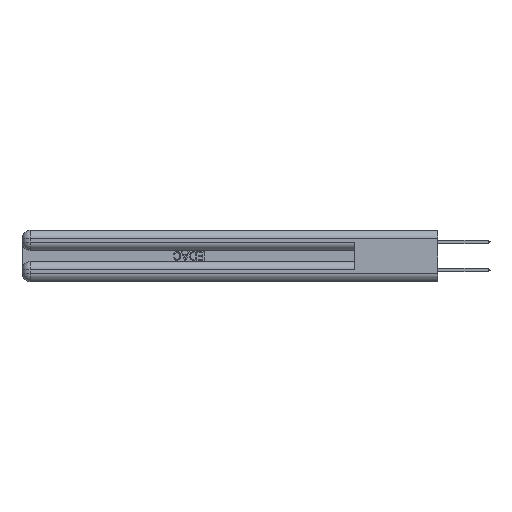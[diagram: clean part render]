
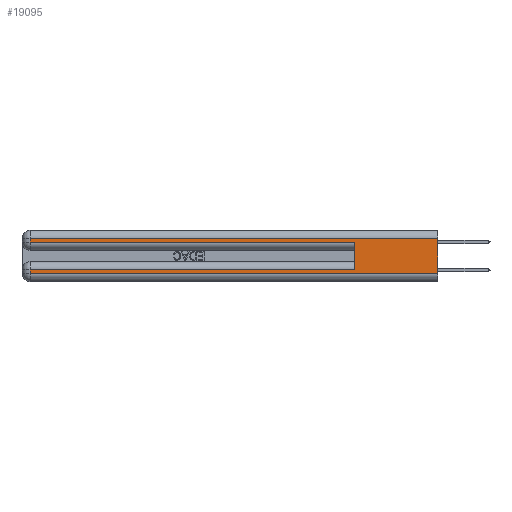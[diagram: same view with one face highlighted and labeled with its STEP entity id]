
A CAD part, left-side view. The second image highlights one B-rep face of the part: STEP entity #19095.
In plain terms, the highlighted planar face has unit normal (-1, 0, 0).
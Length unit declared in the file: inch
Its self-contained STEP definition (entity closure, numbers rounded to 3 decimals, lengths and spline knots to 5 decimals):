
#151 = DIRECTION ( 'NONE',  ( 0., -1., 0. ) ) ;
#419 = ORIENTED_EDGE ( 'NONE', *, *, #30161, .T. ) ;
#722 = LINE ( 'NONE', #13140, #3649 ) ;
#1049 = ORIENTED_EDGE ( 'NONE', *, *, #32594, .T. ) ;
#2635 = ORIENTED_EDGE ( 'NONE', *, *, #19150, .F. ) ;
#3004 = CARTESIAN_POINT ( 'NONE',  ( 0., 0.6, 0.285 ) ) ;
#3334 = EDGE_CURVE ( 'NONE', #20882, #11685, #32982, .T. ) ;
#3649 = VECTOR ( 'NONE', #11130, 39.37008 ) ;
#4140 = DIRECTION ( 'NONE',  ( 1., 0., 0. ) ) ;
#4533 = VERTEX_POINT ( 'NONE', #5880 ) ;
#5880 = CARTESIAN_POINT ( 'NONE',  ( 0., 0., 0.31 ) ) ;
#6239 = DIRECTION ( 'NONE',  ( 0., 0., -1. ) ) ;
#7169 = ORIENTED_EDGE ( 'NONE', *, *, #36159, .F. ) ;
#7286 = DIRECTION ( 'NONE',  ( 0., 1., 0. ) ) ;
#7424 = AXIS2_PLACEMENT_3D ( 'NONE', #38414, #4140, #38285 ) ;
#7446 = LINE ( 'NONE', #11478, #27318 ) ;
#8128 = VERTEX_POINT ( 'NONE', #12417 ) ;
#9615 = VERTEX_POINT ( 'NONE', #18670 ) ;
#10002 = CARTESIAN_POINT ( 'NONE',  ( 0., 0., 0.31 ) ) ;
#11044 = VERTEX_POINT ( 'NONE', #37557 ) ;
#11130 = DIRECTION ( 'NONE',  ( 0., 0., -1. ) ) ;
#11478 = CARTESIAN_POINT ( 'NONE',  ( 0., 0., 0.37 ) ) ;
#11680 = VECTOR ( 'NONE', #20246, 39.37008 ) ;
#11685 = VERTEX_POINT ( 'NONE', #35344 ) ;
#11845 = CARTESIAN_POINT ( 'NONE',  ( 0., 0., 0.06 ) ) ;
#12417 = CARTESIAN_POINT ( 'NONE',  ( 0., 2.94, 0.285 ) ) ;
#13140 = CARTESIAN_POINT ( 'NONE',  ( 0., 2.94, 0.37 ) ) ;
#14024 = DIRECTION ( 'NONE',  ( 0., -1., 0. ) ) ;
#14092 = VECTOR ( 'NONE', #6239, 39.37008 ) ;
#14095 = LINE ( 'NONE', #32731, #11680 ) ;
#15074 = LINE ( 'NONE', #24683, #25749 ) ;
#15416 = EDGE_CURVE ( 'NONE', #9615, #20882, #16678, .T. ) ;
#15979 = VECTOR ( 'NONE', #14024, 39.37008 ) ;
#16678 = LINE ( 'NONE', #37232, #18129 ) ;
#16850 = VECTOR ( 'NONE', #7286, 39.37008 ) ;
#17681 = EDGE_CURVE ( 'NONE', #11685, #26953, #20354, .T. ) ;
#18129 = VECTOR ( 'NONE', #18644, 39.37008 ) ;
#18644 = DIRECTION ( 'NONE',  ( 0., 1., 0. ) ) ;
#18670 = CARTESIAN_POINT ( 'NONE',  ( 0., 0.6, 0.085 ) ) ;
#18800 = LINE ( 'NONE', #10002, #16850 ) ;
#19095 = ADVANCED_FACE ( 'NONE', ( #29655 ), #22978, .F. ) ;
#19150 = EDGE_CURVE ( 'NONE', #9615, #19434, #14095, .T. ) ;
#19434 = VERTEX_POINT ( 'NONE', #3004 ) ;
#20246 = DIRECTION ( 'NONE',  ( 0., 0., 1. ) ) ;
#20354 = LINE ( 'NONE', #11845, #15979 ) ;
#20882 = VERTEX_POINT ( 'NONE', #32548 ) ;
#22978 = PLANE ( 'NONE',  #7424 ) ;
#23848 = CARTESIAN_POINT ( 'NONE',  ( 0., 0., 0.06 ) ) ;
#24683 = CARTESIAN_POINT ( 'NONE',  ( 0., 0., 0.285 ) ) ;
#24793 = CARTESIAN_POINT ( 'NONE',  ( 0., 2.94, 0.37 ) ) ;
#25749 = VECTOR ( 'NONE', #151, 39.37008 ) ;
#26317 = EDGE_CURVE ( 'NONE', #8128, #19434, #15074, .T. ) ;
#26953 = VERTEX_POINT ( 'NONE', #23848 ) ;
#27318 = VECTOR ( 'NONE', #33419, 39.37008 ) ;
#29655 = FACE_OUTER_BOUND ( 'NONE', #39906, .T. ) ;
#30161 = EDGE_CURVE ( 'NONE', #11044, #8128, #722, .T. ) ;
#31949 = ORIENTED_EDGE ( 'NONE', *, *, #26317, .T. ) ;
#32548 = CARTESIAN_POINT ( 'NONE',  ( 0., 2.94, 0.085 ) ) ;
#32594 = EDGE_CURVE ( 'NONE', #4533, #11044, #18800, .T. ) ;
#32731 = CARTESIAN_POINT ( 'NONE',  ( 0., 0.6, 0.145 ) ) ;
#32982 = LINE ( 'NONE', #24793, #14092 ) ;
#33264 = ORIENTED_EDGE ( 'NONE', *, *, #17681, .T. ) ;
#33419 = DIRECTION ( 'NONE',  ( 0., 0., -1. ) ) ;
#34525 = ORIENTED_EDGE ( 'NONE', *, *, #3334, .T. ) ;
#35344 = CARTESIAN_POINT ( 'NONE',  ( 0., 2.94, 0.06 ) ) ;
#36159 = EDGE_CURVE ( 'NONE', #4533, #26953, #7446, .T. ) ;
#37232 = CARTESIAN_POINT ( 'NONE',  ( 0., 0., 0.085 ) ) ;
#37557 = CARTESIAN_POINT ( 'NONE',  ( 0., 2.94, 0.31 ) ) ;
#38285 = DIRECTION ( 'NONE',  ( 0., 0., -1. ) ) ;
#38414 = CARTESIAN_POINT ( 'NONE',  ( 0., 0., 0.37 ) ) ;
#38736 = ORIENTED_EDGE ( 'NONE', *, *, #15416, .T. ) ;
#39906 = EDGE_LOOP ( 'NONE', ( #7169, #1049, #419, #31949, #2635, #38736, #34525, #33264 ) ) ;
